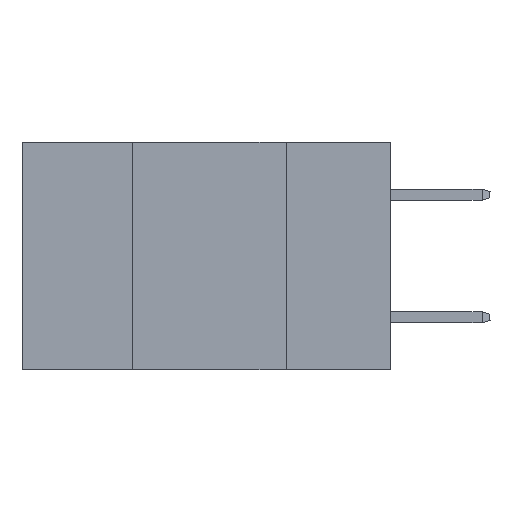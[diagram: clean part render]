
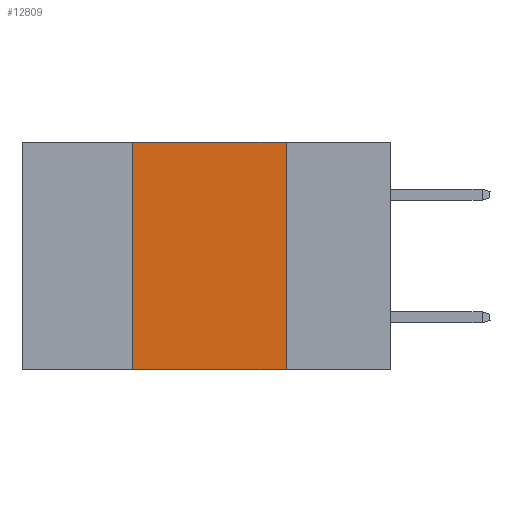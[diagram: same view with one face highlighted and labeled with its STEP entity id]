
A CAD part, left-side view. The second image highlights one B-rep face of the part: STEP entity #12809.
In plain terms, the highlighted planar face has unit normal (-1, 0, 0).
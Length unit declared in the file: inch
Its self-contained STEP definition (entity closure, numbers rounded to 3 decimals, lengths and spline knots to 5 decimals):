
#56 = VERTEX_POINT ( 'NONE', #3898 ) ;
#673 = EDGE_CURVE ( 'NONE', #6630, #4768, #12485, .T. ) ;
#1682 = CARTESIAN_POINT ( 'NONE',  ( 0., 0.17, 0. ) ) ;
#2391 = VECTOR ( 'NONE', #11497, 39.37008 ) ;
#3841 = CARTESIAN_POINT ( 'NONE',  ( 0., 0.6, -0.37 ) ) ;
#3898 = CARTESIAN_POINT ( 'NONE',  ( 0., 0.17, 0. ) ) ;
#4068 = CARTESIAN_POINT ( 'NONE',  ( 0., 0.42, 0. ) ) ;
#4322 = EDGE_LOOP ( 'NONE', ( #7239, #10752, #7644, #11170 ) ) ;
#4554 = DIRECTION ( 'NONE',  ( 1., 0., 0. ) ) ;
#4768 = VERTEX_POINT ( 'NONE', #16234 ) ;
#5366 = VECTOR ( 'NONE', #17134, 39.37008 ) ;
#5587 = CARTESIAN_POINT ( 'NONE',  ( 0., 0.42, -0.37 ) ) ;
#5694 = CARTESIAN_POINT ( 'NONE',  ( 0., 0.17, -0.37 ) ) ;
#5993 = FACE_OUTER_BOUND ( 'NONE', #4322, .T. ) ;
#6160 = CARTESIAN_POINT ( 'NONE',  ( 0., 0.6, 0. ) ) ;
#6630 = VERTEX_POINT ( 'NONE', #5587 ) ;
#6754 = AXIS2_PLACEMENT_3D ( 'NONE', #12569, #4554, #13898 ) ;
#7180 = DIRECTION ( 'NONE',  ( 0., 0., -1. ) ) ;
#7239 = ORIENTED_EDGE ( 'NONE', *, *, #11549, .F. ) ;
#7644 = ORIENTED_EDGE ( 'NONE', *, *, #673, .F. ) ;
#8439 = EDGE_CURVE ( 'NONE', #6630, #13926, #16445, .T. ) ;
#8538 = PLANE ( 'NONE',  #6754 ) ;
#9358 = VECTOR ( 'NONE', #17220, 39.37008 ) ;
#10752 = ORIENTED_EDGE ( 'NONE', *, *, #17096, .F. ) ;
#11030 = LINE ( 'NONE', #1682, #14178 ) ;
#11170 = ORIENTED_EDGE ( 'NONE', *, *, #8439, .T. ) ;
#11497 = DIRECTION ( 'NONE',  ( 0., -1., 0. ) ) ;
#11549 = EDGE_CURVE ( 'NONE', #56, #13926, #11030, .T. ) ;
#12485 = LINE ( 'NONE', #4068, #5366 ) ;
#12569 = CARTESIAN_POINT ( 'NONE',  ( 0., 0.6, 0. ) ) ;
#12809 = ADVANCED_FACE ( 'NONE', ( #5993 ), #8538, .F. ) ;
#13167 = LINE ( 'NONE', #6160, #2391 ) ;
#13898 = DIRECTION ( 'NONE',  ( 0., 0., -1. ) ) ;
#13926 = VERTEX_POINT ( 'NONE', #5694 ) ;
#14178 = VECTOR ( 'NONE', #7180, 39.37008 ) ;
#16234 = CARTESIAN_POINT ( 'NONE',  ( 0., 0.42, 0. ) ) ;
#16445 = LINE ( 'NONE', #3841, #9358 ) ;
#17096 = EDGE_CURVE ( 'NONE', #4768, #56, #13167, .T. ) ;
#17134 = DIRECTION ( 'NONE',  ( 0., 0., 1. ) ) ;
#17220 = DIRECTION ( 'NONE',  ( 0., -1., 0. ) ) ;
